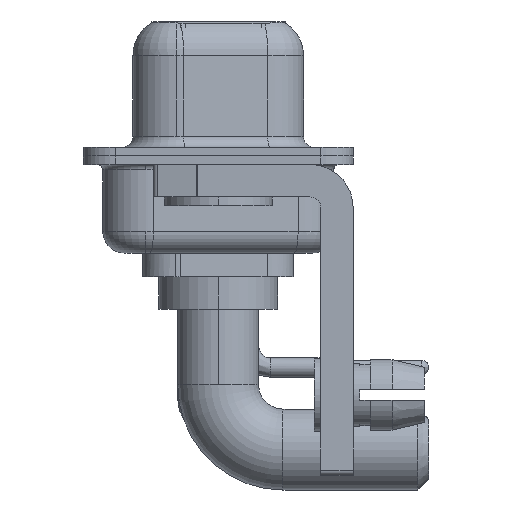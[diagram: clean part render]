
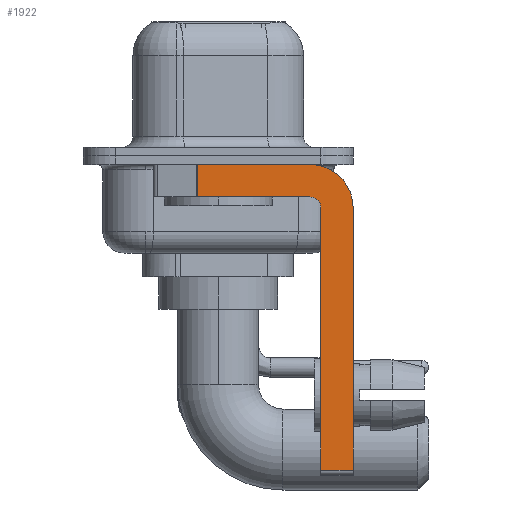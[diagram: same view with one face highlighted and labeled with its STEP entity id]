
A CAD part, left-side view. The second image highlights one B-rep face of the part: STEP entity #1922.
In plain terms, the highlighted planar face has unit normal (-1, 0, 0).
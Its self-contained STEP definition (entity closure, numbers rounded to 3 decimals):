
#49 = EDGE_LOOP ( 'NONE', ( #19672, #3624, #3658, #13759, #11157, #21268, #9027, #466 ) ) ;
#252 = VERTEX_POINT ( 'NONE', #8689 ) ;
#466 = ORIENTED_EDGE ( 'NONE', *, *, #16770, .F. ) ;
#1297 = EDGE_CURVE ( 'NONE', #9933, #7684, #21968, .T. ) ;
#1922 = ADVANCED_FACE ( 'NONE', ( #12906 ), #5256, .F. ) ;
#2273 = CIRCLE ( 'NONE', #19226, 2. ) ;
#2936 = DIRECTION ( 'NONE',  ( 0., 0., 1. ) ) ;
#3624 = ORIENTED_EDGE ( 'NONE', *, *, #11707, .T. ) ;
#3658 = ORIENTED_EDGE ( 'NONE', *, *, #19519, .F. ) ;
#4497 = VERTEX_POINT ( 'NONE', #16259 ) ;
#5137 = DIRECTION ( 'NONE',  ( 1., 0., 0. ) ) ;
#5256 = PLANE ( 'NONE',  #5655 ) ;
#5348 = DIRECTION ( 'NONE',  ( 0., -1., 0. ) ) ;
#5389 = DIRECTION ( 'NONE',  ( -1., 0., 0. ) ) ;
#5655 = AXIS2_PLACEMENT_3D ( 'NONE', #22035, #5137, #18461 ) ;
#5991 = CARTESIAN_POINT ( 'NONE',  ( -2.9, -4.75, -14.55 ) ) ;
#6457 = CARTESIAN_POINT ( 'NONE',  ( -2.9, 3., -0.4 ) ) ;
#6844 = VECTOR ( 'NONE', #17597, 1000. ) ;
#6860 = VECTOR ( 'NONE', #5348, 1000. ) ;
#7684 = VERTEX_POINT ( 'NONE', #18807 ) ;
#7869 = VERTEX_POINT ( 'NONE', #16470 ) ;
#8454 = LINE ( 'NONE', #6457, #12909 ) ;
#8689 = CARTESIAN_POINT ( 'NONE',  ( -2.9, -4.25, -1.9 ) ) ;
#8704 = DIRECTION ( 'NONE',  ( 0., -1., 0. ) ) ;
#8941 = LINE ( 'NONE', #14613, #6860 ) ;
#9027 = ORIENTED_EDGE ( 'NONE', *, *, #20604, .F. ) ;
#9202 = LINE ( 'NONE', #14755, #24065 ) ;
#9435 = CARTESIAN_POINT ( 'NONE',  ( -2.9, -4.25, -2.4 ) ) ;
#9559 = EDGE_CURVE ( 'NONE', #7684, #252, #13709, .T. ) ;
#9933 = VERTEX_POINT ( 'NONE', #5991 ) ;
#10056 = CARTESIAN_POINT ( 'NONE',  ( -2.9, 0.978, -1.9 ) ) ;
#10797 = DIRECTION ( 'NONE',  ( 0., 0., -1. ) ) ;
#11157 = ORIENTED_EDGE ( 'NONE', *, *, #1297, .F. ) ;
#11621 = CARTESIAN_POINT ( 'NONE',  ( -2.9, 0.978, -0.4 ) ) ;
#11707 = EDGE_CURVE ( 'NONE', #16748, #18714, #16336, .T. ) ;
#11785 = VECTOR ( 'NONE', #18201, 1000. ) ;
#12906 = FACE_OUTER_BOUND ( 'NONE', #49, .T. ) ;
#12909 = VECTOR ( 'NONE', #8704, 1000. ) ;
#13483 = EDGE_CURVE ( 'NONE', #9933, #4497, #8941, .T. ) ;
#13709 = CIRCLE ( 'NONE', #19623, 0.5 ) ;
#13759 = ORIENTED_EDGE ( 'NONE', *, *, #9559, .F. ) ;
#14613 = CARTESIAN_POINT ( 'NONE',  ( -2.9, -4.25, -14.55 ) ) ;
#14703 = VECTOR ( 'NONE', #18029, 1000. ) ;
#14755 = CARTESIAN_POINT ( 'NONE',  ( -2.9, -6.25, -2.4 ) ) ;
#16259 = CARTESIAN_POINT ( 'NONE',  ( -2.9, -6.25, -14.55 ) ) ;
#16336 = LINE ( 'NONE', #10056, #6844 ) ;
#16389 = CARTESIAN_POINT ( 'NONE',  ( -2.9, -4.25, -2.4 ) ) ;
#16406 = EDGE_CURVE ( 'NONE', #16748, #19102, #8454, .T. ) ;
#16470 = CARTESIAN_POINT ( 'NONE',  ( -2.9, -6.25, -2.4 ) ) ;
#16476 = CARTESIAN_POINT ( 'NONE',  ( -2.9, -4.25, -1.9 ) ) ;
#16748 = VERTEX_POINT ( 'NONE', #11621 ) ;
#16770 = EDGE_CURVE ( 'NONE', #19102, #7869, #2273, .T. ) ;
#17074 = DIRECTION ( 'NONE',  ( 1., 0., 0. ) ) ;
#17597 = DIRECTION ( 'NONE',  ( 0., 0., -1. ) ) ;
#18029 = DIRECTION ( 'NONE',  ( 0., 0., 1. ) ) ;
#18201 = DIRECTION ( 'NONE',  ( 0., 1., 0. ) ) ;
#18461 = DIRECTION ( 'NONE',  ( 0., 0., -1. ) ) ;
#18714 = VERTEX_POINT ( 'NONE', #20475 ) ;
#18807 = CARTESIAN_POINT ( 'NONE',  ( -2.9, -4.75, -2.4 ) ) ;
#19102 = VERTEX_POINT ( 'NONE', #21926 ) ;
#19161 = DIRECTION ( 'NONE',  ( 0., 0., -1. ) ) ;
#19226 = AXIS2_PLACEMENT_3D ( 'NONE', #9435, #17074, #19161 ) ;
#19519 = EDGE_CURVE ( 'NONE', #252, #18714, #22019, .T. ) ;
#19623 = AXIS2_PLACEMENT_3D ( 'NONE', #16389, #5389, #2936 ) ;
#19672 = ORIENTED_EDGE ( 'NONE', *, *, #16406, .F. ) ;
#20475 = CARTESIAN_POINT ( 'NONE',  ( -2.9, 0.978, -1.9 ) ) ;
#20604 = EDGE_CURVE ( 'NONE', #7869, #4497, #9202, .T. ) ;
#21268 = ORIENTED_EDGE ( 'NONE', *, *, #13483, .T. ) ;
#21847 = CARTESIAN_POINT ( 'NONE',  ( -2.9, -4.75, -14.8 ) ) ;
#21926 = CARTESIAN_POINT ( 'NONE',  ( -2.9, -4.25, -0.4 ) ) ;
#21968 = LINE ( 'NONE', #21847, #14703 ) ;
#22019 = LINE ( 'NONE', #16476, #11785 ) ;
#22035 = CARTESIAN_POINT ( 'NONE',  ( -2.9, -4.25, -2.4 ) ) ;
#24065 = VECTOR ( 'NONE', #10797, 1000. ) ;
